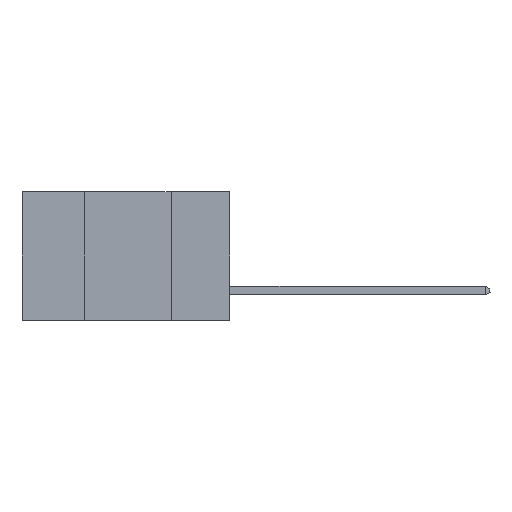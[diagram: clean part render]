
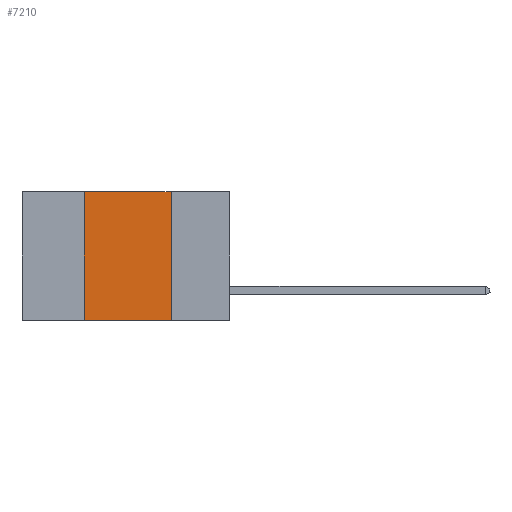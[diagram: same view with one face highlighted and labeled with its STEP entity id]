
A CAD part, left-side view. The second image highlights one B-rep face of the part: STEP entity #7210.
In plain terms, the highlighted planar face has unit normal (-1, 0, 0).
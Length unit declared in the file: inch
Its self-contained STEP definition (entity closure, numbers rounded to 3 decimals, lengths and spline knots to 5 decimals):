
#973 = VERTEX_POINT ( 'NONE', #9899 ) ;
#1279 = VERTEX_POINT ( 'NONE', #4034 ) ;
#1403 = VERTEX_POINT ( 'NONE', #5321 ) ;
#1425 = VECTOR ( 'NONE', #6904, 39.37008 ) ;
#2146 = CARTESIAN_POINT ( 'NONE',  ( 0., 0.6, 0. ) ) ;
#2278 = VECTOR ( 'NONE', #9958, 39.37008 ) ;
#2300 = DIRECTION ( 'NONE',  ( 1., 0., 0. ) ) ;
#2485 = EDGE_CURVE ( 'NONE', #1403, #7568, #8568, .T. ) ;
#2801 = DIRECTION ( 'NONE',  ( 0., -1., 0. ) ) ;
#2903 = ORIENTED_EDGE ( 'NONE', *, *, #2485, .F. ) ;
#3204 = EDGE_CURVE ( 'NONE', #973, #1279, #7579, .T. ) ;
#3369 = ORIENTED_EDGE ( 'NONE', *, *, #4201, .F. ) ;
#3617 = AXIS2_PLACEMENT_3D ( 'NONE', #2146, #2300, #8352 ) ;
#3930 = LINE ( 'NONE', #5085, #1425 ) ;
#4034 = CARTESIAN_POINT ( 'NONE',  ( 0., 0.17, -0.37 ) ) ;
#4201 = EDGE_CURVE ( 'NONE', #7568, #973, #3930, .T. ) ;
#4565 = EDGE_CURVE ( 'NONE', #1403, #1279, #9329, .T. ) ;
#5085 = CARTESIAN_POINT ( 'NONE',  ( 0., 0.6, 0. ) ) ;
#5110 = VECTOR ( 'NONE', #10592, 39.37008 ) ;
#5321 = CARTESIAN_POINT ( 'NONE',  ( 0., 0.42, -0.37 ) ) ;
#5342 = CARTESIAN_POINT ( 'NONE',  ( 0., 0.42, 0. ) ) ;
#6904 = DIRECTION ( 'NONE',  ( 0., -1., 0. ) ) ;
#7121 = VECTOR ( 'NONE', #2801, 39.37008 ) ;
#7210 = ADVANCED_FACE ( 'NONE', ( #8695 ), #8457, .F. ) ;
#7494 = EDGE_LOOP ( 'NONE', ( #11110, #3369, #2903, #7804 ) ) ;
#7568 = VERTEX_POINT ( 'NONE', #7739 ) ;
#7579 = LINE ( 'NONE', #9053, #2278 ) ;
#7739 = CARTESIAN_POINT ( 'NONE',  ( 0., 0.42, 0. ) ) ;
#7804 = ORIENTED_EDGE ( 'NONE', *, *, #4565, .T. ) ;
#8352 = DIRECTION ( 'NONE',  ( 0., 0., -1. ) ) ;
#8457 = PLANE ( 'NONE',  #3617 ) ;
#8568 = LINE ( 'NONE', #5342, #5110 ) ;
#8695 = FACE_OUTER_BOUND ( 'NONE', #7494, .T. ) ;
#9053 = CARTESIAN_POINT ( 'NONE',  ( 0., 0.17, 0. ) ) ;
#9059 = CARTESIAN_POINT ( 'NONE',  ( 0., 0.6, -0.37 ) ) ;
#9329 = LINE ( 'NONE', #9059, #7121 ) ;
#9899 = CARTESIAN_POINT ( 'NONE',  ( 0., 0.17, 0. ) ) ;
#9958 = DIRECTION ( 'NONE',  ( 0., 0., -1. ) ) ;
#10592 = DIRECTION ( 'NONE',  ( 0., 0., 1. ) ) ;
#11110 = ORIENTED_EDGE ( 'NONE', *, *, #3204, .F. ) ;
